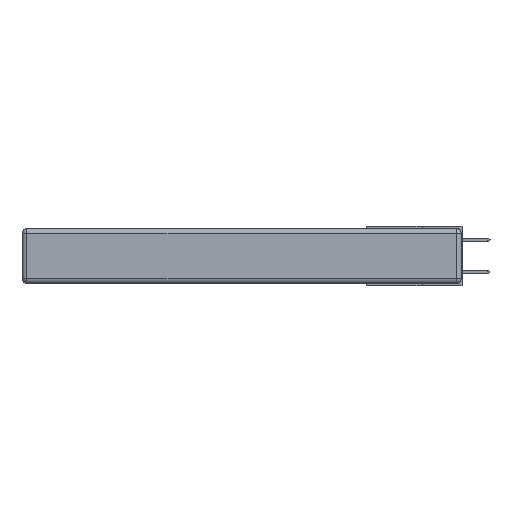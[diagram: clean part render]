
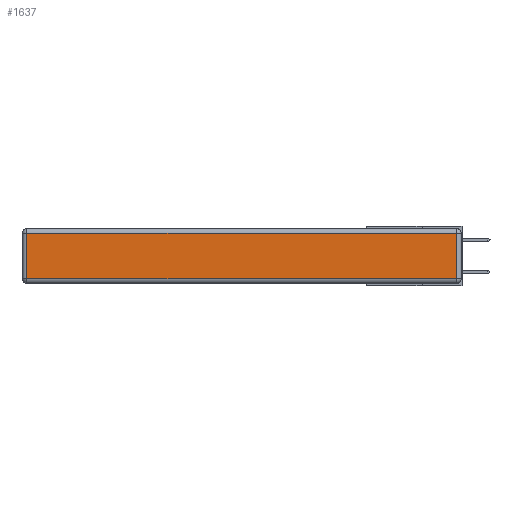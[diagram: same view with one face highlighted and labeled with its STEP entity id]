
A CAD part, left-side view. The second image highlights one B-rep face of the part: STEP entity #1637.
In plain terms, the highlighted planar face has unit normal (-1, 0, 0).
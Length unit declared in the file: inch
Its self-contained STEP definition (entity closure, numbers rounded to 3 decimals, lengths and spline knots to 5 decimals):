
#912 = VECTOR ( 'NONE', #10496, 39.37008 ) ;
#959 = VERTEX_POINT ( 'NONE', #25568 ) ;
#1637 = ADVANCED_FACE ( 'NONE', ( #13546 ), #14983, .T. ) ;
#3121 = EDGE_CURVE ( 'NONE', #9077, #22646, #18360, .T. ) ;
#5807 = CARTESIAN_POINT ( 'NONE',  ( 0., 2.72, -0.03 ) ) ;
#5957 = VERTEX_POINT ( 'NONE', #5807 ) ;
#6681 = EDGE_CURVE ( 'NONE', #22646, #959, #18810, .T. ) ;
#9077 = VERTEX_POINT ( 'NONE', #14845 ) ;
#9799 = DIRECTION ( 'NONE',  ( 0., 0., 1. ) ) ;
#10496 = DIRECTION ( 'NONE',  ( 0., 1., 0. ) ) ;
#11109 = CARTESIAN_POINT ( 'NONE',  ( 0., 0., -0.313 ) ) ;
#11513 = LINE ( 'NONE', #20415, #912 ) ;
#11853 = CARTESIAN_POINT ( 'NONE',  ( 0., 0.03, -0.313 ) ) ;
#13080 = VECTOR ( 'NONE', #15082, 39.37008 ) ;
#13546 = FACE_OUTER_BOUND ( 'NONE', #14046, .T. ) ;
#13677 = LINE ( 'NONE', #23179, #21724 ) ;
#13884 = CARTESIAN_POINT ( 'NONE',  ( 0., 0., -0.343 ) ) ;
#14000 = ORIENTED_EDGE ( 'NONE', *, *, #3121, .T. ) ;
#14046 = EDGE_LOOP ( 'NONE', ( #14000, #17548, #14601, #18736 ) ) ;
#14601 = ORIENTED_EDGE ( 'NONE', *, *, #23818, .T. ) ;
#14845 = CARTESIAN_POINT ( 'NONE',  ( 0., 2.72, -0.313 ) ) ;
#14983 = PLANE ( 'NONE',  #23382 ) ;
#15082 = DIRECTION ( 'NONE',  ( 0., -1., 0. ) ) ;
#16207 = EDGE_CURVE ( 'NONE', #5957, #9077, #13677, .T. ) ;
#17262 = VECTOR ( 'NONE', #24236, 39.37008 ) ;
#17438 = DIRECTION ( 'NONE',  ( 0., 0., -1. ) ) ;
#17548 = ORIENTED_EDGE ( 'NONE', *, *, #6681, .T. ) ;
#18360 = LINE ( 'NONE', #11109, #13080 ) ;
#18736 = ORIENTED_EDGE ( 'NONE', *, *, #16207, .T. ) ;
#18810 = LINE ( 'NONE', #21977, #17262 ) ;
#19725 = DIRECTION ( 'NONE',  ( -1., 0., 0. ) ) ;
#20415 = CARTESIAN_POINT ( 'NONE',  ( 0., 2.75, -0.03 ) ) ;
#21724 = VECTOR ( 'NONE', #17438, 39.37008 ) ;
#21977 = CARTESIAN_POINT ( 'NONE',  ( 0., 0.03, -0.343 ) ) ;
#22646 = VERTEX_POINT ( 'NONE', #11853 ) ;
#23179 = CARTESIAN_POINT ( 'NONE',  ( 0., 2.72, -0.343 ) ) ;
#23382 = AXIS2_PLACEMENT_3D ( 'NONE', #13884, #19725, #9799 ) ;
#23818 = EDGE_CURVE ( 'NONE', #959, #5957, #11513, .T. ) ;
#24236 = DIRECTION ( 'NONE',  ( 0., 0., 1. ) ) ;
#25568 = CARTESIAN_POINT ( 'NONE',  ( 0., 0.03, -0.03 ) ) ;
